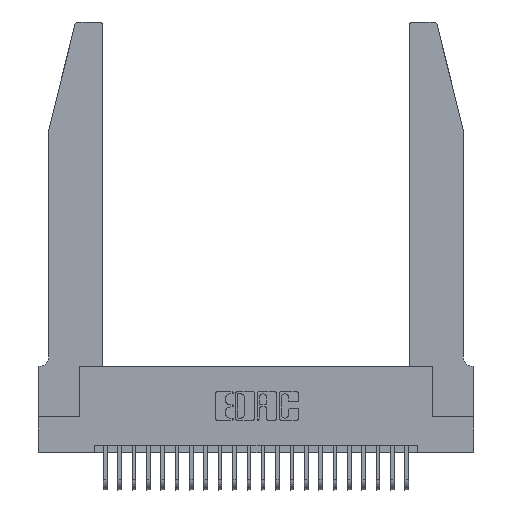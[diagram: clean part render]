
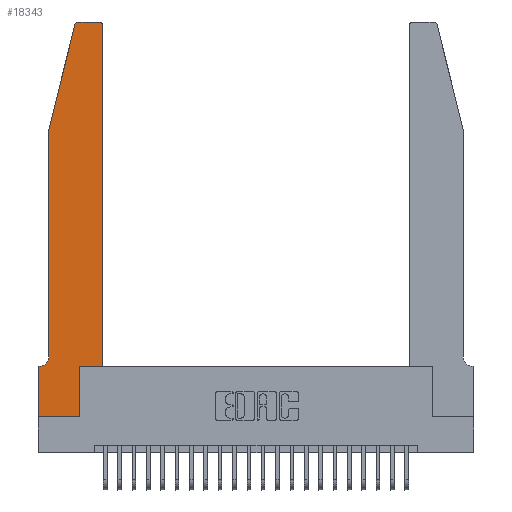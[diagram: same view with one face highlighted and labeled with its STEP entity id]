
A CAD part, top view. The second image highlights one B-rep face of the part: STEP entity #18343.
In plain terms, the highlighted planar face has unit normal (0, 0, 1).
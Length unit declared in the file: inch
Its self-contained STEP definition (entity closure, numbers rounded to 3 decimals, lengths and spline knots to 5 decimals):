
#81 = CARTESIAN_POINT ( 'NONE',  ( 0.0755, 0.35, 0.37 ) ) ;
#87 = LINE ( 'NONE', #8579, #21438 ) ;
#196 = EDGE_LOOP ( 'NONE', ( #16989, #6235, #2288, #15012, #16293, #25387, #6259, #9359, #2142, #10407, #9472, #16004 ) ) ;
#354 = DIRECTION ( 'NONE',  ( 0., -1., 0. ) ) ;
#498 = EDGE_CURVE ( 'NONE', #14347, #15216, #16404, .T. ) ;
#580 = VECTOR ( 'NONE', #19740, 39.37008 ) ;
#851 = DIRECTION ( 'NONE',  ( 0., 0., 1. ) ) ;
#919 = VERTEX_POINT ( 'NONE', #18057 ) ;
#1405 = EDGE_CURVE ( 'NONE', #12002, #20385, #3301, .T. ) ;
#1442 = VECTOR ( 'NONE', #7996, 39.37008 ) ;
#1491 = EDGE_CURVE ( 'NONE', #20385, #24212, #16995, .T. ) ;
#1641 = VECTOR ( 'NONE', #21155, 39.37008 ) ;
#2083 = DIRECTION ( 'NONE',  ( 0., 0., 1. ) ) ;
#2142 = ORIENTED_EDGE ( 'NONE', *, *, #22136, .T. ) ;
#2229 = AXIS2_PLACEMENT_3D ( 'NONE', #4248, #18666, #14554 ) ;
#2288 = ORIENTED_EDGE ( 'NONE', *, *, #25126, .T. ) ;
#2637 = CARTESIAN_POINT ( 'NONE',  ( 0.0055, 0.35, 0.37 ) ) ;
#3301 = LINE ( 'NONE', #14746, #14114 ) ;
#3972 = AXIS2_PLACEMENT_3D ( 'NONE', #16258, #2083, #22416 ) ;
#4092 = DIRECTION ( 'NONE',  ( 0., -1., 0. ) ) ;
#4188 = CARTESIAN_POINT ( 'NONE',  ( 0.4205, 2.75, 0.37 ) ) ;
#4248 = CARTESIAN_POINT ( 'NONE',  ( 0., 0.35, 0.37 ) ) ;
#4309 = LINE ( 'NONE', #7944, #14175 ) ;
#4799 = CARTESIAN_POINT ( 'NONE',  ( 0., 0., 0.37 ) ) ;
#5575 = CIRCLE ( 'NONE', #3972, 0.03 ) ;
#5955 = CARTESIAN_POINT ( 'NONE',  ( 0., 0., 0.37 ) ) ;
#6235 = ORIENTED_EDGE ( 'NONE', *, *, #25769, .T. ) ;
#6259 = ORIENTED_EDGE ( 'NONE', *, *, #1405, .T. ) ;
#7345 = EDGE_CURVE ( 'NONE', #18359, #15754, #25618, .T. ) ;
#7627 = CARTESIAN_POINT ( 'NONE',  ( 0.2865, 0.35, 0.37 ) ) ;
#7944 = CARTESIAN_POINT ( 'NONE',  ( 0.0755, 2., 0.37 ) ) ;
#7996 = DIRECTION ( 'NONE',  ( 0., 1., 0. ) ) ;
#8114 = VERTEX_POINT ( 'NONE', #7627 ) ;
#8146 = AXIS2_PLACEMENT_3D ( 'NONE', #12855, #851, #21243 ) ;
#8579 = CARTESIAN_POINT ( 'NONE',  ( 0.0755, 2., 0.37 ) ) ;
#9359 = ORIENTED_EDGE ( 'NONE', *, *, #1491, .T. ) ;
#9472 = ORIENTED_EDGE ( 'NONE', *, *, #498, .T. ) ;
#9633 = CIRCLE ( 'NONE', #8146, 0.03 ) ;
#10103 = CARTESIAN_POINT ( 'NONE',  ( 0.284, 2.75, 0.37 ) ) ;
#10157 = LINE ( 'NONE', #19571, #580 ) ;
#10407 = ORIENTED_EDGE ( 'NONE', *, *, #21991, .T. ) ;
#11626 = VERTEX_POINT ( 'NONE', #4188 ) ;
#11909 = CARTESIAN_POINT ( 'NONE',  ( 0.2865, 0.35, 0.37 ) ) ;
#11970 = CARTESIAN_POINT ( 'NONE',  ( 0.25487, 2.72718, 0.37 ) ) ;
#12002 = VERTEX_POINT ( 'NONE', #13583 ) ;
#12156 = DIRECTION ( 'NONE',  ( 0., 1., 0. ) ) ;
#12173 = EDGE_CURVE ( 'NONE', #15216, #11626, #5575, .T. ) ;
#12353 = CARTESIAN_POINT ( 'NONE',  ( 0.2605, 2.75, 0.37 ) ) ;
#12521 = VERTEX_POINT ( 'NONE', #11970 ) ;
#12855 = CARTESIAN_POINT ( 'NONE',  ( 0.284, 2.72, 0.37 ) ) ;
#13003 = FACE_OUTER_BOUND ( 'NONE', #196, .T. ) ;
#13319 = DIRECTION ( 'NONE',  ( 0., 0., -1. ) ) ;
#13583 = CARTESIAN_POINT ( 'NONE',  ( 0., 0.35, 0.37 ) ) ;
#13755 = LINE ( 'NONE', #81, #15342 ) ;
#13776 = VERTEX_POINT ( 'NONE', #10103 ) ;
#14114 = VECTOR ( 'NONE', #354, 39.37008 ) ;
#14175 = VECTOR ( 'NONE', #4092, 39.37008 ) ;
#14347 = VERTEX_POINT ( 'NONE', #23608 ) ;
#14554 = DIRECTION ( 'NONE',  ( 1., 0., 0. ) ) ;
#14677 = DIRECTION ( 'NONE',  ( -0.239, -0.971, 0. ) ) ;
#14746 = CARTESIAN_POINT ( 'NONE',  ( 0., 0., 0.37 ) ) ;
#15012 = ORIENTED_EDGE ( 'NONE', *, *, #23505, .T. ) ;
#15216 = VERTEX_POINT ( 'NONE', #23939 ) ;
#15342 = VECTOR ( 'NONE', #20369, 39.37008 ) ;
#15678 = CARTESIAN_POINT ( 'NONE',  ( 0.0055, 0.42, 0.37 ) ) ;
#15754 = VERTEX_POINT ( 'NONE', #2637 ) ;
#16004 = ORIENTED_EDGE ( 'NONE', *, *, #12173, .T. ) ;
#16199 = VECTOR ( 'NONE', #12156, 39.37008 ) ;
#16258 = CARTESIAN_POINT ( 'NONE',  ( 0.4205, 2.72, 0.37 ) ) ;
#16293 = ORIENTED_EDGE ( 'NONE', *, *, #7345, .T. ) ;
#16404 = LINE ( 'NONE', #20183, #1442 ) ;
#16443 = CARTESIAN_POINT ( 'NONE',  ( 0.0755, 0.42, 0.37 ) ) ;
#16625 = EDGE_CURVE ( 'NONE', #11626, #13776, #24646, .T. ) ;
#16828 = LINE ( 'NONE', #11909, #16199 ) ;
#16989 = ORIENTED_EDGE ( 'NONE', *, *, #16625, .T. ) ;
#16995 = LINE ( 'NONE', #5955, #26246 ) ;
#18057 = CARTESIAN_POINT ( 'NONE',  ( 0.0755, 2., 0.37 ) ) ;
#18343 = ADVANCED_FACE ( 'NONE', ( #13003 ), #20451, .T. ) ;
#18359 = VERTEX_POINT ( 'NONE', #16443 ) ;
#18666 = DIRECTION ( 'NONE',  ( 0., 0., 1. ) ) ;
#18825 = DIRECTION ( 'NONE',  ( 1., 0., 0. ) ) ;
#19571 = CARTESIAN_POINT ( 'NONE',  ( 0.4505, 0.35, 0.37 ) ) ;
#19740 = DIRECTION ( 'NONE',  ( 1., 0., 0. ) ) ;
#20183 = CARTESIAN_POINT ( 'NONE',  ( 0.4505, 0.35, 0.37 ) ) ;
#20369 = DIRECTION ( 'NONE',  ( -1., 0., 0. ) ) ;
#20385 = VERTEX_POINT ( 'NONE', #4799 ) ;
#20451 = PLANE ( 'NONE',  #2229 ) ;
#20925 = DIRECTION ( 'NONE',  ( -1., 0., 0. ) ) ;
#21155 = DIRECTION ( 'NONE',  ( -1., 0., 0. ) ) ;
#21243 = DIRECTION ( 'NONE',  ( 1., 0., 0. ) ) ;
#21438 = VECTOR ( 'NONE', #14677, 39.37008 ) ;
#21991 = EDGE_CURVE ( 'NONE', #8114, #14347, #10157, .T. ) ;
#22136 = EDGE_CURVE ( 'NONE', #24212, #8114, #16828, .T. ) ;
#22416 = DIRECTION ( 'NONE',  ( 1., 0., 0. ) ) ;
#22517 = AXIS2_PLACEMENT_3D ( 'NONE', #15678, #13319, #20925 ) ;
#23505 = EDGE_CURVE ( 'NONE', #919, #18359, #4309, .T. ) ;
#23608 = CARTESIAN_POINT ( 'NONE',  ( 0.4505, 0.35, 0.37 ) ) ;
#23939 = CARTESIAN_POINT ( 'NONE',  ( 0.4505, 2.72, 0.37 ) ) ;
#24212 = VERTEX_POINT ( 'NONE', #24470 ) ;
#24470 = CARTESIAN_POINT ( 'NONE',  ( 0.2865, 0., 0.37 ) ) ;
#24646 = LINE ( 'NONE', #12353, #1641 ) ;
#25126 = EDGE_CURVE ( 'NONE', #12521, #919, #87, .T. ) ;
#25387 = ORIENTED_EDGE ( 'NONE', *, *, #25483, .T. ) ;
#25483 = EDGE_CURVE ( 'NONE', #15754, #12002, #13755, .T. ) ;
#25618 = CIRCLE ( 'NONE', #22517, 0.07 ) ;
#25769 = EDGE_CURVE ( 'NONE', #13776, #12521, #9633, .T. ) ;
#26246 = VECTOR ( 'NONE', #18825, 39.37008 ) ;
